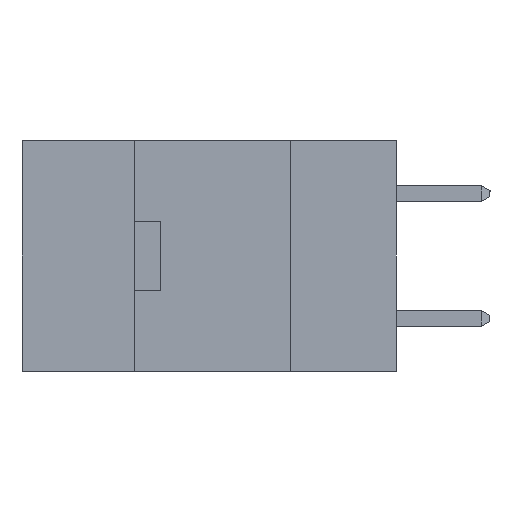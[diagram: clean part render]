
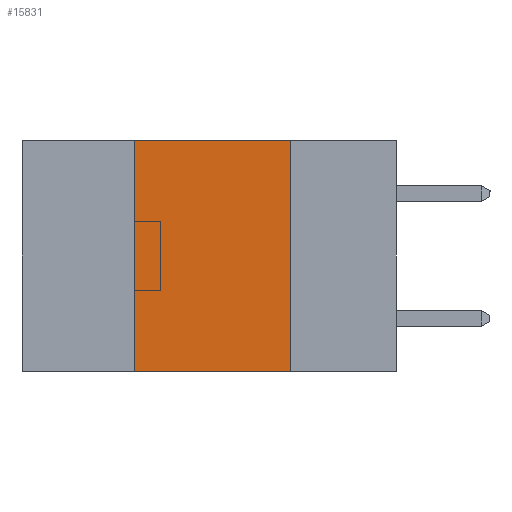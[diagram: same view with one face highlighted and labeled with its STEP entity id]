
A CAD part, left-side view. The second image highlights one B-rep face of the part: STEP entity #15831.
In plain terms, the highlighted planar face has unit normal (-1, 0, 0).
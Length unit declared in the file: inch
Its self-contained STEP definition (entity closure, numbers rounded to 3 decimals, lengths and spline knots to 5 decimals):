
#27 = DIRECTION ( 'NONE',  ( 0., -1., 0. ) ) ;
#168 = CARTESIAN_POINT ( 'NONE',  ( 0., 0.6, 0. ) ) ;
#691 = EDGE_CURVE ( 'NONE', #11913, #17665, #25513, .T. ) ;
#2848 = CARTESIAN_POINT ( 'NONE',  ( 0., 0.17, -0.37 ) ) ;
#3276 = ORIENTED_EDGE ( 'NONE', *, *, #691, .F. ) ;
#3861 = EDGE_CURVE ( 'NONE', #13515, #7882, #13290, .T. ) ;
#4432 = ORIENTED_EDGE ( 'NONE', *, *, #3861, .F. ) ;
#4743 = PLANE ( 'NONE',  #17838 ) ;
#5755 = DIRECTION ( 'NONE',  ( 0., 0., -1. ) ) ;
#6503 = CARTESIAN_POINT ( 'NONE',  ( 0., 0.6, 0. ) ) ;
#6788 = CARTESIAN_POINT ( 'NONE',  ( 0., 0.42, -0.37 ) ) ;
#7882 = VERTEX_POINT ( 'NONE', #22193 ) ;
#8369 = LINE ( 'NONE', #19762, #10002 ) ;
#10002 = VECTOR ( 'NONE', #27, 39.37008 ) ;
#11913 = VERTEX_POINT ( 'NONE', #21508 ) ;
#12102 = EDGE_CURVE ( 'NONE', #7882, #11913, #19783, .T. ) ;
#12192 = VECTOR ( 'NONE', #22365, 39.37008 ) ;
#13290 = LINE ( 'NONE', #6788, #12192 ) ;
#13321 = ORIENTED_EDGE ( 'NONE', *, *, #15653, .T. ) ;
#13515 = VERTEX_POINT ( 'NONE', #15054 ) ;
#14168 = VECTOR ( 'NONE', #5755, 39.37008 ) ;
#15054 = CARTESIAN_POINT ( 'NONE',  ( 0., 0.42, -0.37 ) ) ;
#15190 = EDGE_LOOP ( 'NONE', ( #3276, #24412, #4432, #13321 ) ) ;
#15653 = EDGE_CURVE ( 'NONE', #13515, #17665, #8369, .T. ) ;
#15831 = ADVANCED_FACE ( 'NONE', ( #26640 ), #4743, .F. ) ;
#17665 = VERTEX_POINT ( 'NONE', #2848 ) ;
#17838 = AXIS2_PLACEMENT_3D ( 'NONE', #168, #22334, #26924 ) ;
#19762 = CARTESIAN_POINT ( 'NONE',  ( 0., 0.6, -0.37 ) ) ;
#19783 = LINE ( 'NONE', #6503, #25895 ) ;
#21508 = CARTESIAN_POINT ( 'NONE',  ( 0., 0.17, 0. ) ) ;
#22193 = CARTESIAN_POINT ( 'NONE',  ( 0., 0.42, 0. ) ) ;
#22334 = DIRECTION ( 'NONE',  ( 1., 0., 0. ) ) ;
#22365 = DIRECTION ( 'NONE',  ( 0., 0., 1. ) ) ;
#24412 = ORIENTED_EDGE ( 'NONE', *, *, #12102, .F. ) ;
#25375 = CARTESIAN_POINT ( 'NONE',  ( 0., 0.17, -0.37 ) ) ;
#25513 = LINE ( 'NONE', #25375, #14168 ) ;
#25895 = VECTOR ( 'NONE', #26249, 39.37008 ) ;
#26249 = DIRECTION ( 'NONE',  ( 0., -1., 0. ) ) ;
#26640 = FACE_OUTER_BOUND ( 'NONE', #15190, .T. ) ;
#26924 = DIRECTION ( 'NONE',  ( 0., 0., -1. ) ) ;
